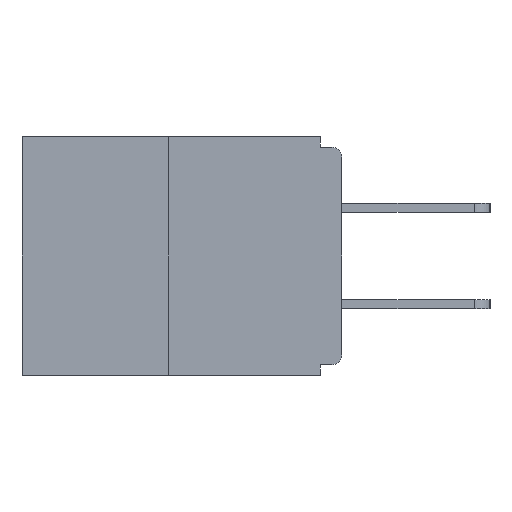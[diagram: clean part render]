
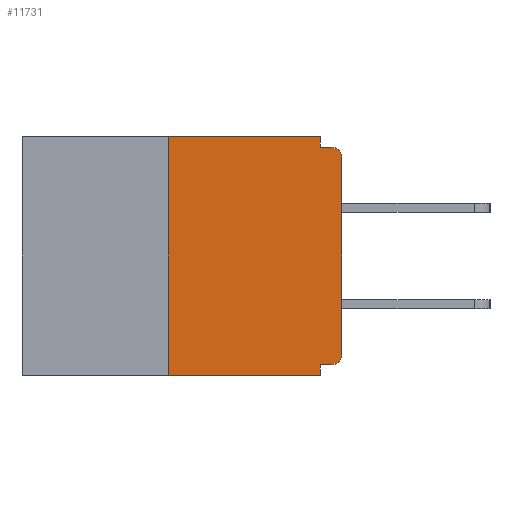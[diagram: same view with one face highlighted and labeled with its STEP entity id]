
A CAD part, left-side view. The second image highlights one B-rep face of the part: STEP entity #11731.
In plain terms, the highlighted planar face has unit normal (-1, 0, 0).
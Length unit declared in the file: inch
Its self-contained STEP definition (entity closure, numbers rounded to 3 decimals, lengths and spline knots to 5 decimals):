
#360 = CARTESIAN_POINT ( 'NONE',  ( 0., 0.25, -0.343 ) ) ;
#465 = EDGE_CURVE ( 'NONE', #15388, #7271, #13441, .T. ) ;
#524 = AXIS2_PLACEMENT_3D ( 'NONE', #5732, #10821, #9586 ) ;
#771 = VERTEX_POINT ( 'NONE', #13754 ) ;
#794 = EDGE_CURVE ( 'NONE', #771, #3471, #4043, .T. ) ;
#869 = DIRECTION ( 'NONE',  ( 0., 0., 1. ) ) ;
#878 = VECTOR ( 'NONE', #14329, 39.37008 ) ;
#909 = VECTOR ( 'NONE', #10849, 39.37008 ) ;
#985 = DIRECTION ( 'NONE',  ( 0., 0., -1. ) ) ;
#1026 = LINE ( 'NONE', #7130, #6422 ) ;
#1173 = CARTESIAN_POINT ( 'NONE',  ( 0., 0.031, -0.015 ) ) ;
#1759 = CARTESIAN_POINT ( 'NONE',  ( 0., 0.015, -0.015 ) ) ;
#1971 = LINE ( 'NONE', #6248, #15347 ) ;
#2291 = LINE ( 'NONE', #15926, #909 ) ;
#2705 = EDGE_CURVE ( 'NONE', #7354, #15388, #1026, .T. ) ;
#2756 = CARTESIAN_POINT ( 'NONE',  ( 0., 0.015, -0.03 ) ) ;
#2769 = CARTESIAN_POINT ( 'NONE',  ( 0., 0.46, 0. ) ) ;
#2931 = ORIENTED_EDGE ( 'NONE', *, *, #8362, .F. ) ;
#3040 = FACE_OUTER_BOUND ( 'NONE', #8195, .T. ) ;
#3180 = CARTESIAN_POINT ( 'NONE',  ( 0., 0., -0.328 ) ) ;
#3471 = VERTEX_POINT ( 'NONE', #12473 ) ;
#3798 = LINE ( 'NONE', #8668, #12602 ) ;
#4006 = AXIS2_PLACEMENT_3D ( 'NONE', #10586, #4080, #4242 ) ;
#4043 = LINE ( 'NONE', #15146, #10459 ) ;
#4080 = DIRECTION ( 'NONE',  ( -1., 0., 0. ) ) ;
#4242 = DIRECTION ( 'NONE',  ( 0., 0., -1. ) ) ;
#4303 = ORIENTED_EDGE ( 'NONE', *, *, #13914, .T. ) ;
#4652 = ORIENTED_EDGE ( 'NONE', *, *, #14017, .T. ) ;
#5085 = ORIENTED_EDGE ( 'NONE', *, *, #2705, .F. ) ;
#5346 = VERTEX_POINT ( 'NONE', #1759 ) ;
#5732 = CARTESIAN_POINT ( 'NONE',  ( 0., 0.46, 0. ) ) ;
#5952 = DIRECTION ( 'NONE',  ( 0., 0., 1. ) ) ;
#6248 = CARTESIAN_POINT ( 'NONE',  ( 0., 0., -0.015 ) ) ;
#6422 = VECTOR ( 'NONE', #869, 39.37008 ) ;
#7130 = CARTESIAN_POINT ( 'NONE',  ( 0., 0.25, 0. ) ) ;
#7271 = VERTEX_POINT ( 'NONE', #11910 ) ;
#7278 = EDGE_CURVE ( 'NONE', #13911, #13071, #12079, .T. ) ;
#7354 = VERTEX_POINT ( 'NONE', #360 ) ;
#7476 = VECTOR ( 'NONE', #10044, 39.37008 ) ;
#7675 = LINE ( 'NONE', #11388, #7476 ) ;
#8195 = EDGE_LOOP ( 'NONE', ( #12795, #5085, #15695, #8243, #2931, #13716, #4652, #4303, #14589, #11026 ) ) ;
#8243 = ORIENTED_EDGE ( 'NONE', *, *, #794, .F. ) ;
#8318 = DIRECTION ( 'NONE',  ( -1., 0., 0. ) ) ;
#8362 = EDGE_CURVE ( 'NONE', #13911, #771, #15169, .T. ) ;
#8668 = CARTESIAN_POINT ( 'NONE',  ( 0., 0., 0. ) ) ;
#8777 = VECTOR ( 'NONE', #10983, 39.37008 ) ;
#8948 = EDGE_CURVE ( 'NONE', #8978, #5346, #1971, .T. ) ;
#8978 = VERTEX_POINT ( 'NONE', #1173 ) ;
#9021 = CARTESIAN_POINT ( 'NONE',  ( 0., 0.015, -0.328 ) ) ;
#9586 = DIRECTION ( 'NONE',  ( 0., 0., -1. ) ) ;
#9625 = CARTESIAN_POINT ( 'NONE',  ( 0., 0., -0.313 ) ) ;
#10044 = DIRECTION ( 'NONE',  ( 0., 0., -1. ) ) ;
#10210 = CIRCLE ( 'NONE', #12734, 0.015 ) ;
#10459 = VECTOR ( 'NONE', #985, 39.37008 ) ;
#10586 = CARTESIAN_POINT ( 'NONE',  ( 0., 0.015, -0.313 ) ) ;
#10821 = DIRECTION ( 'NONE',  ( 1., 0., 0. ) ) ;
#10849 = DIRECTION ( 'NONE',  ( 0., -1., 0. ) ) ;
#10976 = EDGE_CURVE ( 'NONE', #7354, #3471, #2291, .T. ) ;
#10983 = DIRECTION ( 'NONE',  ( 0., 1., 0. ) ) ;
#11026 = ORIENTED_EDGE ( 'NONE', *, *, #11562, .F. ) ;
#11388 = CARTESIAN_POINT ( 'NONE',  ( 0., 0.031, 0. ) ) ;
#11562 = EDGE_CURVE ( 'NONE', #7271, #8978, #7675, .T. ) ;
#11731 = ADVANCED_FACE ( 'NONE', ( #3040 ), #12045, .F. ) ;
#11910 = CARTESIAN_POINT ( 'NONE',  ( 0., 0.031, 0. ) ) ;
#12030 = CARTESIAN_POINT ( 'NONE',  ( 0., 0.25, 0. ) ) ;
#12045 = PLANE ( 'NONE',  #524 ) ;
#12079 = CIRCLE ( 'NONE', #4006, 0.015 ) ;
#12360 = VERTEX_POINT ( 'NONE', #14449 ) ;
#12473 = CARTESIAN_POINT ( 'NONE',  ( 0., 0.031, -0.343 ) ) ;
#12602 = VECTOR ( 'NONE', #5952, 39.37008 ) ;
#12734 = AXIS2_PLACEMENT_3D ( 'NONE', #2756, #8318, #14683 ) ;
#12795 = ORIENTED_EDGE ( 'NONE', *, *, #465, .F. ) ;
#13071 = VERTEX_POINT ( 'NONE', #9625 ) ;
#13441 = LINE ( 'NONE', #2769, #878 ) ;
#13716 = ORIENTED_EDGE ( 'NONE', *, *, #7278, .T. ) ;
#13754 = CARTESIAN_POINT ( 'NONE',  ( 0., 0.031, -0.328 ) ) ;
#13897 = DIRECTION ( 'NONE',  ( 0., -1., 0. ) ) ;
#13911 = VERTEX_POINT ( 'NONE', #9021 ) ;
#13914 = EDGE_CURVE ( 'NONE', #12360, #5346, #10210, .T. ) ;
#14017 = EDGE_CURVE ( 'NONE', #13071, #12360, #3798, .T. ) ;
#14329 = DIRECTION ( 'NONE',  ( 0., -1., 0. ) ) ;
#14449 = CARTESIAN_POINT ( 'NONE',  ( 0., 0., -0.03 ) ) ;
#14589 = ORIENTED_EDGE ( 'NONE', *, *, #8948, .F. ) ;
#14683 = DIRECTION ( 'NONE',  ( 0., 0., -1. ) ) ;
#15146 = CARTESIAN_POINT ( 'NONE',  ( 0., 0.031, -0.343 ) ) ;
#15169 = LINE ( 'NONE', #3180, #8777 ) ;
#15347 = VECTOR ( 'NONE', #13897, 39.37008 ) ;
#15388 = VERTEX_POINT ( 'NONE', #12030 ) ;
#15695 = ORIENTED_EDGE ( 'NONE', *, *, #10976, .T. ) ;
#15926 = CARTESIAN_POINT ( 'NONE',  ( 0., 0.46, -0.343 ) ) ;
